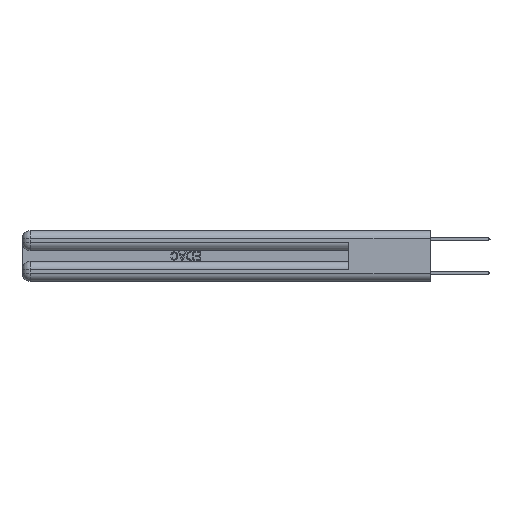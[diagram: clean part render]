
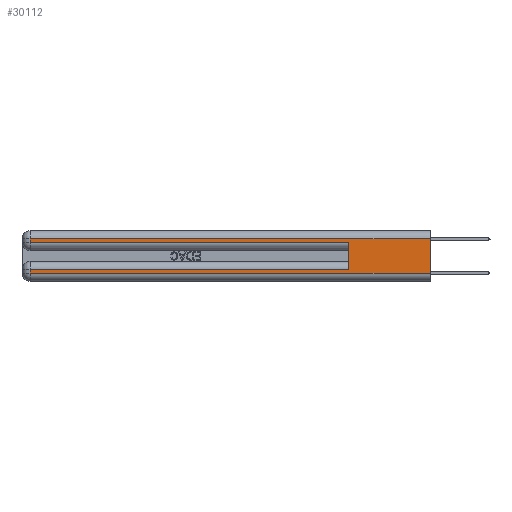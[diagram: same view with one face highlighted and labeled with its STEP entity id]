
A CAD part, left-side view. The second image highlights one B-rep face of the part: STEP entity #30112.
In plain terms, the highlighted planar face has unit normal (-1, 0, 0).
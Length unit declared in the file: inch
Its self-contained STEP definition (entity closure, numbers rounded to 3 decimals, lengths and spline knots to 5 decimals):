
#353 = EDGE_CURVE ( 'NONE', #10128, #8353, #35327, .T. ) ;
#1083 = VERTEX_POINT ( 'NONE', #1742 ) ;
#1181 = CARTESIAN_POINT ( 'NONE',  ( 0., 2.94, 0.31 ) ) ;
#1742 = CARTESIAN_POINT ( 'NONE',  ( 0., 0.6, 0.085 ) ) ;
#2206 = VECTOR ( 'NONE', #3470, 39.37008 ) ;
#2300 = DIRECTION ( 'NONE',  ( 0., -1., 0. ) ) ;
#2807 = LINE ( 'NONE', #2973, #4589 ) ;
#2973 = CARTESIAN_POINT ( 'NONE',  ( 0., 0., 0.085 ) ) ;
#3470 = DIRECTION ( 'NONE',  ( 0., 0., -1. ) ) ;
#3486 = LINE ( 'NONE', #14539, #2206 ) ;
#3625 = DIRECTION ( 'NONE',  ( 0., 0., -1. ) ) ;
#4589 = VECTOR ( 'NONE', #36209, 39.37008 ) ;
#4764 = CARTESIAN_POINT ( 'NONE',  ( 0., 0.6, 0.285 ) ) ;
#4849 = ORIENTED_EDGE ( 'NONE', *, *, #30655, .T. ) ;
#4882 = AXIS2_PLACEMENT_3D ( 'NONE', #5963, #8760, #3625 ) ;
#5209 = CARTESIAN_POINT ( 'NONE',  ( 0., 2.94, 0.06 ) ) ;
#5963 = CARTESIAN_POINT ( 'NONE',  ( 0., 0., 0.37 ) ) ;
#6117 = EDGE_CURVE ( 'NONE', #1083, #35916, #15407, .T. ) ;
#6252 = CARTESIAN_POINT ( 'NONE',  ( 0., 0.6, 0.145 ) ) ;
#7669 = CARTESIAN_POINT ( 'NONE',  ( 0., 2.94, 0.37 ) ) ;
#7671 = VERTEX_POINT ( 'NONE', #10423 ) ;
#7736 = ORIENTED_EDGE ( 'NONE', *, *, #6117, .F. ) ;
#8353 = VERTEX_POINT ( 'NONE', #31161 ) ;
#8760 = DIRECTION ( 'NONE',  ( 1., 0., 0. ) ) ;
#9109 = ORIENTED_EDGE ( 'NONE', *, *, #9557, .T. ) ;
#9557 = EDGE_CURVE ( 'NONE', #7671, #25300, #12305, .T. ) ;
#10128 = VERTEX_POINT ( 'NONE', #5209 ) ;
#10423 = CARTESIAN_POINT ( 'NONE',  ( 0., 0., 0.31 ) ) ;
#12305 = LINE ( 'NONE', #15137, #30658 ) ;
#12716 = ORIENTED_EDGE ( 'NONE', *, *, #27576, .T. ) ;
#12988 = VECTOR ( 'NONE', #22772, 39.37008 ) ;
#13050 = ORIENTED_EDGE ( 'NONE', *, *, #15159, .T. ) ;
#13113 = CARTESIAN_POINT ( 'NONE',  ( 0., 2.94, 0.085 ) ) ;
#14539 = CARTESIAN_POINT ( 'NONE',  ( 0., 2.94, 0.37 ) ) ;
#14636 = VECTOR ( 'NONE', #36102, 39.37008 ) ;
#14671 = LINE ( 'NONE', #28661, #25189 ) ;
#15137 = CARTESIAN_POINT ( 'NONE',  ( 0., 0., 0.31 ) ) ;
#15159 = EDGE_CURVE ( 'NONE', #25300, #16464, #31279, .T. ) ;
#15407 = LINE ( 'NONE', #6252, #17146 ) ;
#16464 = VERTEX_POINT ( 'NONE', #32856 ) ;
#17146 = VECTOR ( 'NONE', #20237, 39.37008 ) ;
#20237 = DIRECTION ( 'NONE',  ( 0., 0., 1. ) ) ;
#21307 = EDGE_CURVE ( 'NONE', #16464, #35916, #31802, .T. ) ;
#22024 = ORIENTED_EDGE ( 'NONE', *, *, #353, .T. ) ;
#22412 = FACE_OUTER_BOUND ( 'NONE', #36183, .T. ) ;
#22571 = CARTESIAN_POINT ( 'NONE',  ( 0., 0., 0.06 ) ) ;
#22772 = DIRECTION ( 'NONE',  ( 0., -1., 0. ) ) ;
#22911 = DIRECTION ( 'NONE',  ( 0., 0., -1. ) ) ;
#24110 = EDGE_CURVE ( 'NONE', #7671, #8353, #14671, .T. ) ;
#24373 = VECTOR ( 'NONE', #2300, 39.37008 ) ;
#25189 = VECTOR ( 'NONE', #22911, 39.37008 ) ;
#25300 = VERTEX_POINT ( 'NONE', #1181 ) ;
#27576 = EDGE_CURVE ( 'NONE', #1083, #34020, #2807, .T. ) ;
#28661 = CARTESIAN_POINT ( 'NONE',  ( 0., 0., 0.37 ) ) ;
#28883 = PLANE ( 'NONE',  #4882 ) ;
#30112 = ADVANCED_FACE ( 'NONE', ( #22412 ), #28883, .F. ) ;
#30379 = CARTESIAN_POINT ( 'NONE',  ( 0., 0., 0.285 ) ) ;
#30655 = EDGE_CURVE ( 'NONE', #34020, #10128, #3486, .T. ) ;
#30658 = VECTOR ( 'NONE', #32018, 39.37008 ) ;
#31161 = CARTESIAN_POINT ( 'NONE',  ( 0., 0., 0.06 ) ) ;
#31279 = LINE ( 'NONE', #7669, #14636 ) ;
#31802 = LINE ( 'NONE', #30379, #24373 ) ;
#32018 = DIRECTION ( 'NONE',  ( 0., 1., 0. ) ) ;
#32856 = CARTESIAN_POINT ( 'NONE',  ( 0., 2.94, 0.285 ) ) ;
#33614 = ORIENTED_EDGE ( 'NONE', *, *, #24110, .F. ) ;
#34020 = VERTEX_POINT ( 'NONE', #13113 ) ;
#34048 = ORIENTED_EDGE ( 'NONE', *, *, #21307, .T. ) ;
#35327 = LINE ( 'NONE', #22571, #12988 ) ;
#35916 = VERTEX_POINT ( 'NONE', #4764 ) ;
#36102 = DIRECTION ( 'NONE',  ( 0., 0., -1. ) ) ;
#36183 = EDGE_LOOP ( 'NONE', ( #33614, #9109, #13050, #34048, #7736, #12716, #4849, #22024 ) ) ;
#36209 = DIRECTION ( 'NONE',  ( 0., 1., 0. ) ) ;
